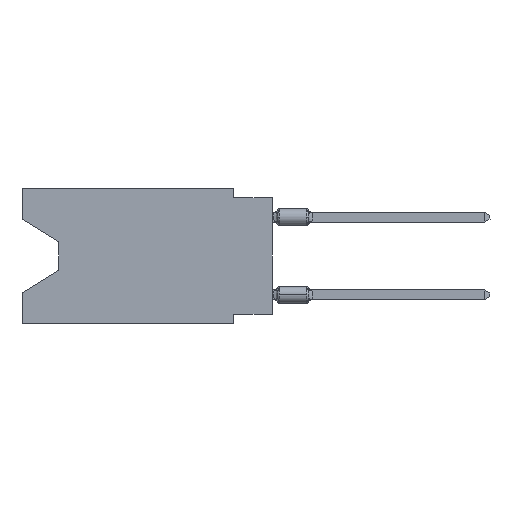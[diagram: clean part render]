
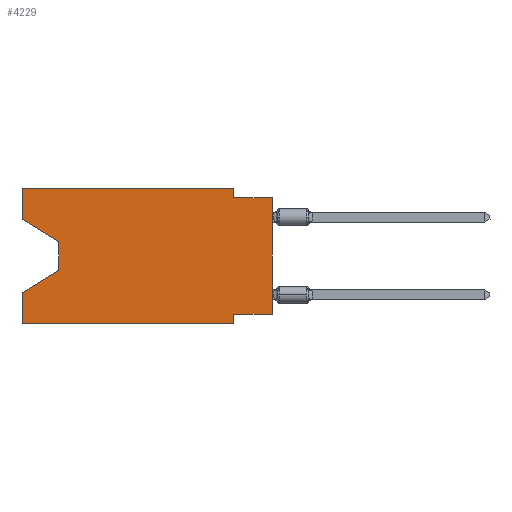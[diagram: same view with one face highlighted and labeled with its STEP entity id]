
A CAD part, left-side view. The second image highlights one B-rep face of the part: STEP entity #4229.
In plain terms, the highlighted planar face has unit normal (-1, 0, 0).
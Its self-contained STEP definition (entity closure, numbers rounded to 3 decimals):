
#450 = CARTESIAN_POINT ( 'NONE',  ( 0., 0., -8.255 ) ) ;
#502 = CARTESIAN_POINT ( 'NONE',  ( 0., 2.54, -8.89 ) ) ;
#701 = ORIENTED_EDGE ( 'NONE', *, *, #10520, .T. ) ;
#728 = AXIS2_PLACEMENT_3D ( 'NONE', #12265, #2017, #11306 ) ;
#1201 = CARTESIAN_POINT ( 'NONE',  ( 0., 13.97, -5.385 ) ) ;
#1527 = VERTEX_POINT ( 'NONE', #5560 ) ;
#1630 = DIRECTION ( 'NONE',  ( 0., -1., 0. ) ) ;
#1637 = DIRECTION ( 'NONE',  ( 0., -1., 0. ) ) ;
#1676 = CARTESIAN_POINT ( 'NONE',  ( 0., 0., 0. ) ) ;
#1968 = EDGE_CURVE ( 'NONE', #6532, #10383, #2574, .T. ) ;
#2017 = DIRECTION ( 'NONE',  ( 1., 0., 0. ) ) ;
#2249 = CARTESIAN_POINT ( 'NONE',  ( 0., 16.383, -2.038 ) ) ;
#2489 = EDGE_CURVE ( 'NONE', #2797, #11059, #5508, .T. ) ;
#2574 = LINE ( 'NONE', #1676, #3458 ) ;
#2715 = DIRECTION ( 'NONE',  ( 0., 1., 0. ) ) ;
#2716 = ORIENTED_EDGE ( 'NONE', *, *, #2489, .F. ) ;
#2797 = VERTEX_POINT ( 'NONE', #4335 ) ;
#3142 = ORIENTED_EDGE ( 'NONE', *, *, #1968, .T. ) ;
#3348 = CARTESIAN_POINT ( 'NONE',  ( 0., 13.97, -5.385 ) ) ;
#3417 = DIRECTION ( 'NONE',  ( 0., 0., 1. ) ) ;
#3458 = VECTOR ( 'NONE', #3609, 1000. ) ;
#3482 = DIRECTION ( 'NONE',  ( 0., 0.855, -0.519 ) ) ;
#3609 = DIRECTION ( 'NONE',  ( 0., 0., 1. ) ) ;
#3626 = VERTEX_POINT ( 'NONE', #5411 ) ;
#4003 = VECTOR ( 'NONE', #10351, 1000. ) ;
#4229 = ADVANCED_FACE ( 'NONE', ( #13286 ), #10229, .F. ) ;
#4278 = CARTESIAN_POINT ( 'NONE',  ( 0., 16.383, 0. ) ) ;
#4335 = CARTESIAN_POINT ( 'NONE',  ( 0., 2.54, -8.255 ) ) ;
#4377 = LINE ( 'NONE', #5790, #6381 ) ;
#4480 = LINE ( 'NONE', #12796, #5082 ) ;
#4644 = VECTOR ( 'NONE', #1637, 1000. ) ;
#4645 = VECTOR ( 'NONE', #4927, 1000. ) ;
#4774 = LINE ( 'NONE', #450, #9660 ) ;
#4863 = LINE ( 'NONE', #11003, #4644 ) ;
#4872 = VECTOR ( 'NONE', #11028, 1000. ) ;
#4925 = EDGE_CURVE ( 'NONE', #12748, #10383, #6837, .T. ) ;
#4927 = DIRECTION ( 'NONE',  ( 0., 0., 1. ) ) ;
#4954 = LINE ( 'NONE', #5992, #4872 ) ;
#5082 = VECTOR ( 'NONE', #9740, 1000. ) ;
#5093 = CARTESIAN_POINT ( 'NONE',  ( 0., 2.54, 0. ) ) ;
#5252 = EDGE_CURVE ( 'NONE', #6532, #2797, #4774, .T. ) ;
#5411 = CARTESIAN_POINT ( 'NONE',  ( 0., 16.383, -6.852 ) ) ;
#5508 = LINE ( 'NONE', #502, #5867 ) ;
#5560 = CARTESIAN_POINT ( 'NONE',  ( 0., 16.383, -8.89 ) ) ;
#5585 = VERTEX_POINT ( 'NONE', #1201 ) ;
#5790 = CARTESIAN_POINT ( 'NONE',  ( 0., 16.383, 0. ) ) ;
#5867 = VECTOR ( 'NONE', #9685, 1000. ) ;
#5992 = CARTESIAN_POINT ( 'NONE',  ( 0., 16.383, -2.038 ) ) ;
#6140 = VECTOR ( 'NONE', #6986, 1000. ) ;
#6381 = VECTOR ( 'NONE', #3417, 1000. ) ;
#6532 = VERTEX_POINT ( 'NONE', #12538 ) ;
#6837 = LINE ( 'NONE', #10997, #8774 ) ;
#6986 = DIRECTION ( 'NONE',  ( 0., 0., -1. ) ) ;
#6995 = EDGE_CURVE ( 'NONE', #12883, #12748, #4480, .T. ) ;
#7196 = ORIENTED_EDGE ( 'NONE', *, *, #7727, .T. ) ;
#7482 = EDGE_CURVE ( 'NONE', #1527, #3626, #9922, .T. ) ;
#7727 = EDGE_CURVE ( 'NONE', #5585, #3626, #8536, .T. ) ;
#7787 = ORIENTED_EDGE ( 'NONE', *, *, #12820, .F. ) ;
#7918 = VECTOR ( 'NONE', #3482, 1000. ) ;
#8061 = ORIENTED_EDGE ( 'NONE', *, *, #10638, .F. ) ;
#8536 = LINE ( 'NONE', #3348, #7918 ) ;
#8602 = EDGE_CURVE ( 'NONE', #1527, #11059, #4863, .T. ) ;
#8719 = CARTESIAN_POINT ( 'NONE',  ( 0., 0., -0.635 ) ) ;
#8774 = VECTOR ( 'NONE', #1630, 1000. ) ;
#9182 = LINE ( 'NONE', #4278, #4003 ) ;
#9401 = ORIENTED_EDGE ( 'NONE', *, *, #4925, .F. ) ;
#9415 = VERTEX_POINT ( 'NONE', #11174 ) ;
#9472 = ORIENTED_EDGE ( 'NONE', *, *, #6995, .F. ) ;
#9660 = VECTOR ( 'NONE', #2715, 1000. ) ;
#9685 = DIRECTION ( 'NONE',  ( 0., 0., -1. ) ) ;
#9740 = DIRECTION ( 'NONE',  ( 0., 0., -1. ) ) ;
#9898 = ORIENTED_EDGE ( 'NONE', *, *, #8602, .T. ) ;
#9922 = LINE ( 'NONE', #10932, #4645 ) ;
#10229 = PLANE ( 'NONE',  #728 ) ;
#10351 = DIRECTION ( 'NONE',  ( 0., -1., 0. ) ) ;
#10383 = VERTEX_POINT ( 'NONE', #8719 ) ;
#10520 = EDGE_CURVE ( 'NONE', #11057, #13284, #4954, .T. ) ;
#10638 = EDGE_CURVE ( 'NONE', #9415, #12883, #9182, .T. ) ;
#10932 = CARTESIAN_POINT ( 'NONE',  ( 0., 16.383, 0. ) ) ;
#10997 = CARTESIAN_POINT ( 'NONE',  ( 0., 0., -0.635 ) ) ;
#11003 = CARTESIAN_POINT ( 'NONE',  ( 0., 16.383, -8.89 ) ) ;
#11028 = DIRECTION ( 'NONE',  ( 0., -0.855, -0.519 ) ) ;
#11057 = VERTEX_POINT ( 'NONE', #2249 ) ;
#11059 = VERTEX_POINT ( 'NONE', #11603 ) ;
#11174 = CARTESIAN_POINT ( 'NONE',  ( 0., 16.383, 0. ) ) ;
#11306 = DIRECTION ( 'NONE',  ( 0., 0., -1. ) ) ;
#11355 = ORIENTED_EDGE ( 'NONE', *, *, #7482, .F. ) ;
#11603 = CARTESIAN_POINT ( 'NONE',  ( 0., 2.54, -8.89 ) ) ;
#11682 = CARTESIAN_POINT ( 'NONE',  ( 0., 2.54, -0.635 ) ) ;
#11969 = CARTESIAN_POINT ( 'NONE',  ( 0., 13.97, -3.505 ) ) ;
#12169 = EDGE_CURVE ( 'NONE', #13284, #5585, #13203, .T. ) ;
#12265 = CARTESIAN_POINT ( 'NONE',  ( 0., 16.383, 0. ) ) ;
#12538 = CARTESIAN_POINT ( 'NONE',  ( 0., 0., -8.255 ) ) ;
#12748 = VERTEX_POINT ( 'NONE', #11682 ) ;
#12755 = ORIENTED_EDGE ( 'NONE', *, *, #12169, .T. ) ;
#12796 = CARTESIAN_POINT ( 'NONE',  ( 0., 2.54, 0. ) ) ;
#12820 = EDGE_CURVE ( 'NONE', #11057, #9415, #4377, .T. ) ;
#12883 = VERTEX_POINT ( 'NONE', #5093 ) ;
#12963 = ORIENTED_EDGE ( 'NONE', *, *, #5252, .F. ) ;
#12977 = EDGE_LOOP ( 'NONE', ( #701, #12755, #7196, #11355, #9898, #2716, #12963, #3142, #9401, #9472, #8061, #7787 ) ) ;
#13203 = LINE ( 'NONE', #11969, #6140 ) ;
#13263 = CARTESIAN_POINT ( 'NONE',  ( 0., 13.97, -3.505 ) ) ;
#13284 = VERTEX_POINT ( 'NONE', #13263 ) ;
#13286 = FACE_OUTER_BOUND ( 'NONE', #12977, .T. ) ;
